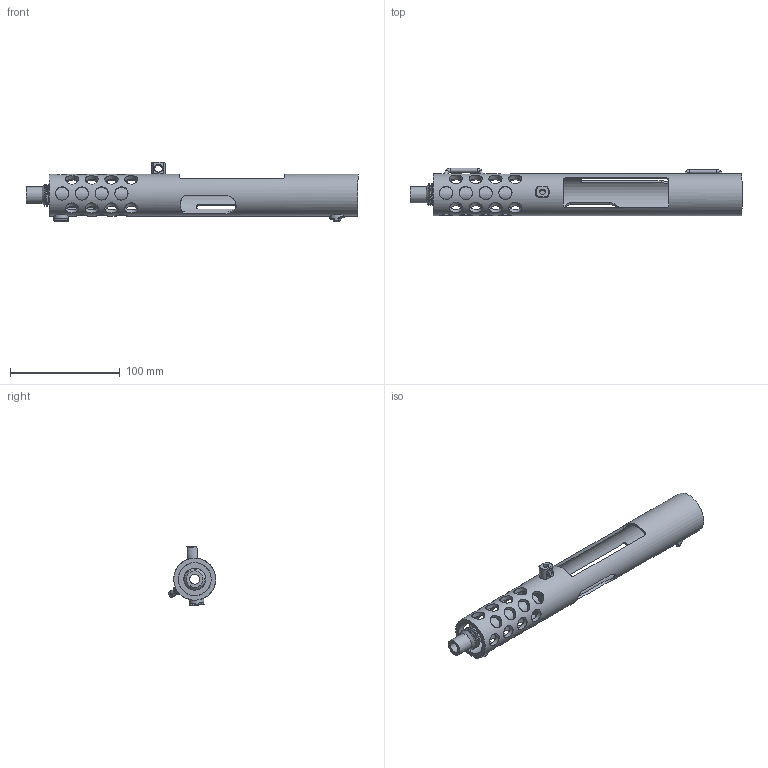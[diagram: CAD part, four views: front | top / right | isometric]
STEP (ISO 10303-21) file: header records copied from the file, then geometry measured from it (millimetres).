
FILE_DESCRIPTION(/* description */ (''),/* implementation_level */ '2;1');
FILE_NAME(/* name */ 'EarlyTec9ButtonSights.step',/* time_stamp */ '2025-06-09T10:47:11-04:00',/* author */ (''),/* organization */ (''),/* preprocessor_version */ 'ST-DEVELOPER v20.1',/* originating_system */ 'Autodesk Translation Framework v14.10.0.0',/* authorisation */ '');
FILE_SCHEMA (('AUTOMOTIVE_DESIGN { 1 0 10303 214 3 1 1 }'));
Length unit declared in the file: millimetre
Products named in the file (1): Mock Up Tec 9
Bounding box: 302.1 x 43.09 x 54.35 mm (x, y, z)
Volume: 75658.1 mm3; surface area: 66074.1 mm2
Topology: 6 solids, 6 shells, 201 faces, 571 edges, 371 vertices
Faces by surface type: cylinder 91, plane 48, bspline 44, torus 11, cone 7
Full cylindrical faces by diameter (mm): 3.5 x6, 5 x2, 7 x1, 8 x1, 9 x2, 12 x31, 13 x2, 15 x2, 16.938 x1, 19.791 x1, 30.1 x1, 34.1 x1, 38.1 x1
Entity records: 12002 total; most frequent: CARTESIAN_POINT 7092, ORIENTED_EDGE 1126, DIRECTION 807, EDGE_CURVE 563, VERTEX_POINT 371, AXIS2_PLACEMENT_3D 332, EDGE_LOOP 274, B_SPLINE_CURVE_WITH_KNOTS 242
